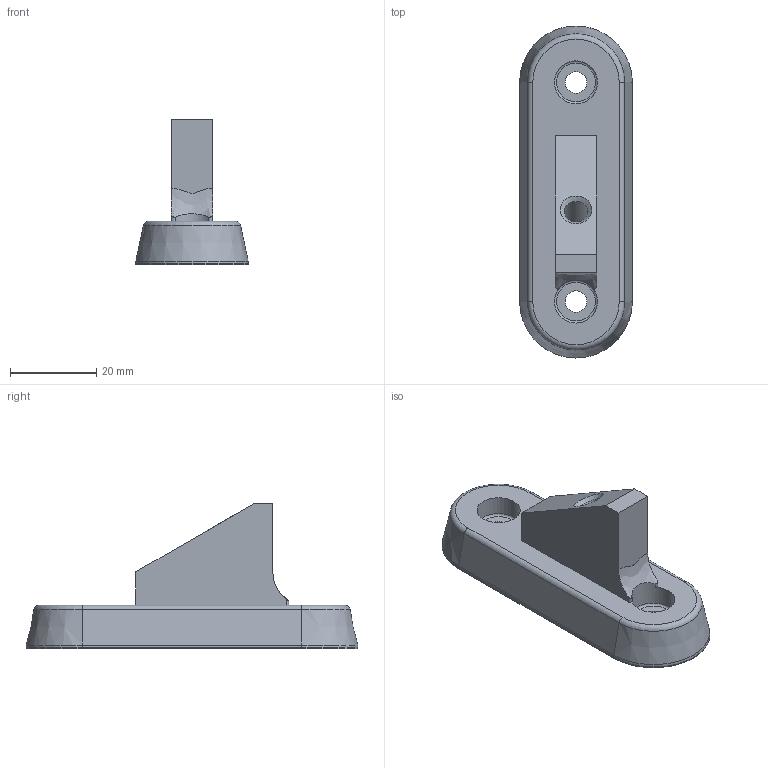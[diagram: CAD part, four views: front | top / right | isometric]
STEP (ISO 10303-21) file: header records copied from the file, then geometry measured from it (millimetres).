
FILE_DESCRIPTION(/* description */ (''),/* implementation_level */ '2;1');
FILE_NAME(/* name */ 'Grip Mount AR15 Based.stp',/* time_stamp */ '2021-10-12T11:17:32-05:00',/* author */ ('johne'),/* organization */ (''),/* preprocessor_version */ 'ST-DEVELOPER v18.1',/* originating_system */ 'Autodesk Inventor 2020',/* authorisation */ '');
FILE_SCHEMA (('AUTOMOTIVE_DESIGN { 1 0 10303 214 3 1 1 }'));
Length unit declared in the file: inch
Products named in the file (1): Grip Mount
Bounding box: 26.16 x 76.96 x 33.7 mm (x, y, z)
Volume: 20411.5 mm3; surface area: 7426.6 mm2
Topology: 1 solids, 1 shells, 38 faces, 96 edges, 61 vertices
Faces by surface type: plane 14, cylinder 13, torus 6, cone 3, bspline 2
Full cylindrical faces by diameter (mm): 5 x2, 5.537 x1, 10 x2
Entity records: 1606 total; most frequent: CARTESIAN_POINT 624, DIRECTION 202, ORIENTED_EDGE 192, EDGE_CURVE 96, AXIS2_PLACEMENT_3D 80, VERTEX_POINT 61, EDGE_LOOP 45, CIRCLE 42
